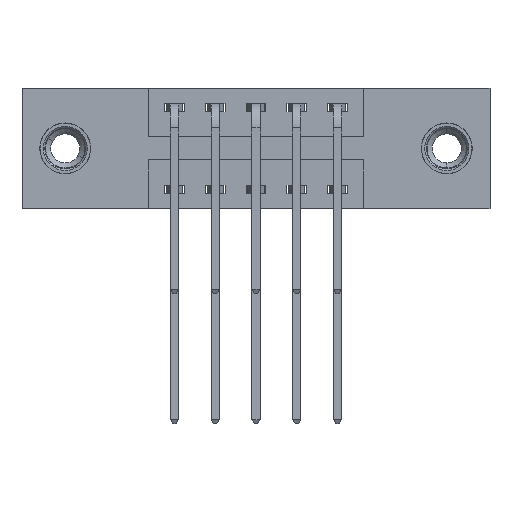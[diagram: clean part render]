
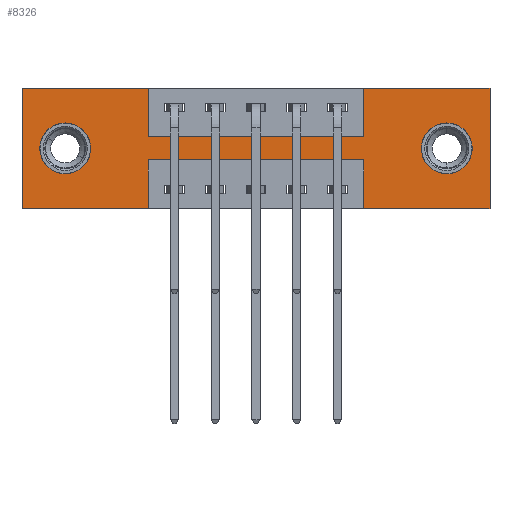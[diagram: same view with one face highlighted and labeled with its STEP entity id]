
A CAD part, front view. The second image highlights one B-rep face of the part: STEP entity #8326.
In plain terms, the highlighted planar face has unit normal (0, -1, 0).
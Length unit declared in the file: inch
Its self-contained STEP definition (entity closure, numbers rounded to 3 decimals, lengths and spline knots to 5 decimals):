
#131 = EDGE_CURVE ( 'NONE', #11071, #2129, #3336, .T. ) ;
#237 = EDGE_CURVE ( 'NONE', #2129, #11071, #4271, .T. ) ;
#284 = VERTEX_POINT ( 'NONE', #6688 ) ;
#333 = LINE ( 'NONE', #10383, #3720 ) ;
#348 = VERTEX_POINT ( 'NONE', #1117 ) ;
#381 = CARTESIAN_POINT ( 'NONE',  ( 1.0475, 0., -0.15 ) ) ;
#484 = FACE_OUTER_BOUND ( 'NONE', #4566, .T. ) ;
#530 = EDGE_CURVE ( 'NONE', #6844, #1163, #3999, .T. ) ;
#602 = DIRECTION ( 'NONE',  ( 1., 0., 0. ) ) ;
#630 = CARTESIAN_POINT ( 'NONE',  ( 0.3875, 0., -0.15 ) ) ;
#813 = CARTESIAN_POINT ( 'NONE',  ( 0.3875, 0., -0.37 ) ) ;
#839 = CARTESIAN_POINT ( 'NONE',  ( 1.435, 0., -0.37 ) ) ;
#855 = DIRECTION ( 'NONE',  ( 1., 0., 0. ) ) ;
#1102 = LINE ( 'NONE', #5677, #9549 ) ;
#1112 = VERTEX_POINT ( 'NONE', #4115 ) ;
#1117 = CARTESIAN_POINT ( 'NONE',  ( 0., 0., 0. ) ) ;
#1163 = VERTEX_POINT ( 'NONE', #7833 ) ;
#1188 = LINE ( 'NONE', #813, #10176 ) ;
#1210 = VERTEX_POINT ( 'NONE', #381 ) ;
#1243 = CARTESIAN_POINT ( 'NONE',  ( 0., 0., 0. ) ) ;
#1629 = DIRECTION ( 'NONE',  ( -1., 0., 0. ) ) ;
#1649 = ORIENTED_EDGE ( 'NONE', *, *, #4094, .F. ) ;
#1797 = CARTESIAN_POINT ( 'NONE',  ( 1.3025, 0., -0.263 ) ) ;
#1811 = CARTESIAN_POINT ( 'NONE',  ( 1.0475, 0., 0. ) ) ;
#1921 = AXIS2_PLACEMENT_3D ( 'NONE', #7068, #6438, #9935 ) ;
#2047 = LINE ( 'NONE', #11222, #11031 ) ;
#2093 = ORIENTED_EDGE ( 'NONE', *, *, #4221, .F. ) ;
#2129 = VERTEX_POINT ( 'NONE', #3947 ) ;
#2257 = VERTEX_POINT ( 'NONE', #4162 ) ;
#2399 = EDGE_CURVE ( 'NONE', #3550, #1112, #7454, .T. ) ;
#2435 = LINE ( 'NONE', #6176, #7049 ) ;
#2518 = CARTESIAN_POINT ( 'NONE',  ( 0.3875, 0., -0.22 ) ) ;
#2685 = ORIENTED_EDGE ( 'NONE', *, *, #530, .F. ) ;
#2696 = VECTOR ( 'NONE', #1629, 39.37008 ) ;
#2750 = VECTOR ( 'NONE', #5591, 39.37008 ) ;
#2811 = CARTESIAN_POINT ( 'NONE',  ( 1.435, 0., 0. ) ) ;
#2924 = CARTESIAN_POINT ( 'NONE',  ( 1.0475, 0., -0.37 ) ) ;
#3074 = CARTESIAN_POINT ( 'NONE',  ( 0.1325, 0., -0.185 ) ) ;
#3094 = AXIS2_PLACEMENT_3D ( 'NONE', #3074, #9155, #3952 ) ;
#3108 = DIRECTION ( 'NONE',  ( -1., 0., 0. ) ) ;
#3163 = VERTEX_POINT ( 'NONE', #10797 ) ;
#3168 = EDGE_CURVE ( 'NONE', #4888, #284, #10099, .T. ) ;
#3336 = CIRCLE ( 'NONE', #1921, 0.078 ) ;
#3488 = VECTOR ( 'NONE', #3922, 39.37008 ) ;
#3535 = VERTEX_POINT ( 'NONE', #839 ) ;
#3550 = VERTEX_POINT ( 'NONE', #1797 ) ;
#3676 = DIRECTION ( 'NONE',  ( 0., -1., 0. ) ) ;
#3684 = LINE ( 'NONE', #8309, #8315 ) ;
#3720 = VECTOR ( 'NONE', #4253, 39.37008 ) ;
#3757 = CARTESIAN_POINT ( 'NONE',  ( 1.3025, 0., -0.185 ) ) ;
#3853 = CARTESIAN_POINT ( 'NONE',  ( 1.435, 0., 0. ) ) ;
#3874 = EDGE_CURVE ( 'NONE', #1163, #5072, #4732, .T. ) ;
#3896 = EDGE_CURVE ( 'NONE', #5072, #4888, #1188, .T. ) ;
#3922 = DIRECTION ( 'NONE',  ( 1., 0., 0. ) ) ;
#3939 = VECTOR ( 'NONE', #9795, 39.37008 ) ;
#3947 = CARTESIAN_POINT ( 'NONE',  ( 0.1325, 0., -0.107 ) ) ;
#3952 = DIRECTION ( 'NONE',  ( 0., 0., 1. ) ) ;
#3957 = AXIS2_PLACEMENT_3D ( 'NONE', #10437, #3676, #7222 ) ;
#3998 = CARTESIAN_POINT ( 'NONE',  ( 0.3875, 0., -0.37 ) ) ;
#3999 = LINE ( 'NONE', #7341, #5464 ) ;
#4094 = EDGE_CURVE ( 'NONE', #1210, #3163, #8289, .T. ) ;
#4115 = CARTESIAN_POINT ( 'NONE',  ( 1.3025, 0., -0.107 ) ) ;
#4162 = CARTESIAN_POINT ( 'NONE',  ( 0.3875, 0., 0. ) ) ;
#4221 = EDGE_CURVE ( 'NONE', #10329, #3535, #6351, .T. ) ;
#4246 = ORIENTED_EDGE ( 'NONE', *, *, #131, .T. ) ;
#4253 = DIRECTION ( 'NONE',  ( 0., 0., -1. ) ) ;
#4268 = ORIENTED_EDGE ( 'NONE', *, *, #5027, .F. ) ;
#4271 = CIRCLE ( 'NONE', #3094, 0.078 ) ;
#4349 = DIRECTION ( 'NONE',  ( 0., 0., -1. ) ) ;
#4545 = ORIENTED_EDGE ( 'NONE', *, *, #9334, .T. ) ;
#4566 = EDGE_LOOP ( 'NONE', ( #6433, #5992, #2685, #4268, #2093, #11196, #1649, #7207, #7860, #8585, #6043, #8374 ) ) ;
#4705 = LINE ( 'NONE', #1243, #3488 ) ;
#4732 = LINE ( 'NONE', #9451, #2696 ) ;
#4888 = VERTEX_POINT ( 'NONE', #3998 ) ;
#5027 = EDGE_CURVE ( 'NONE', #3535, #6844, #3684, .T. ) ;
#5072 = VERTEX_POINT ( 'NONE', #2518 ) ;
#5174 = EDGE_LOOP ( 'NONE', ( #6749, #4246 ) ) ;
#5179 = EDGE_CURVE ( 'NONE', #6739, #1210, #2435, .T. ) ;
#5464 = VECTOR ( 'NONE', #10844, 39.37008 ) ;
#5586 = ORIENTED_EDGE ( 'NONE', *, *, #2399, .T. ) ;
#5591 = DIRECTION ( 'NONE',  ( -1., 0., 0. ) ) ;
#5677 = CARTESIAN_POINT ( 'NONE',  ( 0., 0., 0. ) ) ;
#5773 = FACE_BOUND ( 'NONE', #5174, .T. ) ;
#5948 = VECTOR ( 'NONE', #7806, 39.37008 ) ;
#5992 = ORIENTED_EDGE ( 'NONE', *, *, #3874, .F. ) ;
#6043 = ORIENTED_EDGE ( 'NONE', *, *, #9660, .F. ) ;
#6176 = CARTESIAN_POINT ( 'NONE',  ( 0.3875, 0., -0.15 ) ) ;
#6351 = LINE ( 'NONE', #2811, #3939 ) ;
#6361 = DIRECTION ( 'NONE',  ( 0., 1., 0. ) ) ;
#6433 = ORIENTED_EDGE ( 'NONE', *, *, #3896, .F. ) ;
#6438 = DIRECTION ( 'NONE',  ( 0., 1., 0. ) ) ;
#6625 = EDGE_CURVE ( 'NONE', #348, #2257, #1102, .T. ) ;
#6688 = CARTESIAN_POINT ( 'NONE',  ( 0., 0., -0.37 ) ) ;
#6739 = VERTEX_POINT ( 'NONE', #630 ) ;
#6749 = ORIENTED_EDGE ( 'NONE', *, *, #237, .T. ) ;
#6844 = VERTEX_POINT ( 'NONE', #2924 ) ;
#6895 = DIRECTION ( 'NONE',  ( 0., 0., -1. ) ) ;
#6931 = PLANE ( 'NONE',  #3957 ) ;
#7034 = CIRCLE ( 'NONE', #9051, 0.078 ) ;
#7049 = VECTOR ( 'NONE', #855, 39.37008 ) ;
#7068 = CARTESIAN_POINT ( 'NONE',  ( 0.1325, 0., -0.185 ) ) ;
#7111 = EDGE_LOOP ( 'NONE', ( #4545, #5586 ) ) ;
#7207 = ORIENTED_EDGE ( 'NONE', *, *, #5179, .F. ) ;
#7213 = EDGE_CURVE ( 'NONE', #3163, #10329, #4705, .T. ) ;
#7222 = DIRECTION ( 'NONE',  ( 0., 0., -1. ) ) ;
#7341 = CARTESIAN_POINT ( 'NONE',  ( 1.0475, 0., -0.37 ) ) ;
#7454 = CIRCLE ( 'NONE', #7598, 0.078 ) ;
#7531 = EDGE_CURVE ( 'NONE', #2257, #6739, #333, .T. ) ;
#7598 = AXIS2_PLACEMENT_3D ( 'NONE', #9508, #10413, #4349 ) ;
#7719 = DIRECTION ( 'NONE',  ( 0., 0., 1. ) ) ;
#7806 = DIRECTION ( 'NONE',  ( 0., 0., 1. ) ) ;
#7833 = CARTESIAN_POINT ( 'NONE',  ( 1.0475, 0., -0.22 ) ) ;
#7860 = ORIENTED_EDGE ( 'NONE', *, *, #7531, .F. ) ;
#8117 = DIRECTION ( 'NONE',  ( 0., 0., -1. ) ) ;
#8198 = CARTESIAN_POINT ( 'NONE',  ( 0., 0., -0.37 ) ) ;
#8289 = LINE ( 'NONE', #1811, #5948 ) ;
#8309 = CARTESIAN_POINT ( 'NONE',  ( 0., 0., -0.37 ) ) ;
#8315 = VECTOR ( 'NONE', #3108, 39.37008 ) ;
#8326 = ADVANCED_FACE ( 'NONE', ( #10259, #5773, #484 ), #6931, .T. ) ;
#8374 = ORIENTED_EDGE ( 'NONE', *, *, #3168, .F. ) ;
#8585 = ORIENTED_EDGE ( 'NONE', *, *, #6625, .F. ) ;
#9051 = AXIS2_PLACEMENT_3D ( 'NONE', #3757, #6361, #8117 ) ;
#9155 = DIRECTION ( 'NONE',  ( 0., 1., 0. ) ) ;
#9334 = EDGE_CURVE ( 'NONE', #1112, #3550, #7034, .T. ) ;
#9451 = CARTESIAN_POINT ( 'NONE',  ( 0.3875, 0., -0.22 ) ) ;
#9508 = CARTESIAN_POINT ( 'NONE',  ( 1.3025, 0., -0.185 ) ) ;
#9549 = VECTOR ( 'NONE', #602, 39.37008 ) ;
#9660 = EDGE_CURVE ( 'NONE', #284, #348, #2047, .T. ) ;
#9795 = DIRECTION ( 'NONE',  ( 0., 0., -1. ) ) ;
#9935 = DIRECTION ( 'NONE',  ( 0., 0., 1. ) ) ;
#10099 = LINE ( 'NONE', #8198, #2750 ) ;
#10176 = VECTOR ( 'NONE', #6895, 39.37008 ) ;
#10259 = FACE_BOUND ( 'NONE', #7111, .T. ) ;
#10329 = VERTEX_POINT ( 'NONE', #3853 ) ;
#10383 = CARTESIAN_POINT ( 'NONE',  ( 0.3875, 0., 0. ) ) ;
#10413 = DIRECTION ( 'NONE',  ( 0., 1., 0. ) ) ;
#10437 = CARTESIAN_POINT ( 'NONE',  ( 0., 0., -0.37 ) ) ;
#10797 = CARTESIAN_POINT ( 'NONE',  ( 1.0475, 0., 0. ) ) ;
#10844 = DIRECTION ( 'NONE',  ( 0., 0., 1. ) ) ;
#11031 = VECTOR ( 'NONE', #7719, 39.37008 ) ;
#11071 = VERTEX_POINT ( 'NONE', #11192 ) ;
#11192 = CARTESIAN_POINT ( 'NONE',  ( 0.1325, 0., -0.263 ) ) ;
#11196 = ORIENTED_EDGE ( 'NONE', *, *, #7213, .F. ) ;
#11222 = CARTESIAN_POINT ( 'NONE',  ( 0., 0., 0. ) ) ;
